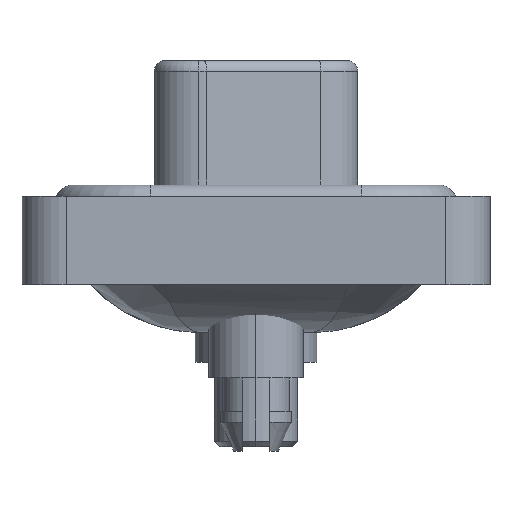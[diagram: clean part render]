
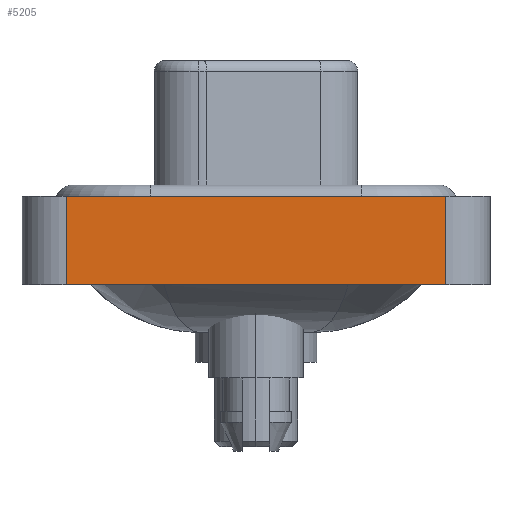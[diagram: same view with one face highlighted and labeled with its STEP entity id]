
A CAD part, left-side view. The second image highlights one B-rep face of the part: STEP entity #5205.
In plain terms, the highlighted planar face has unit normal (-1, 0, 0).
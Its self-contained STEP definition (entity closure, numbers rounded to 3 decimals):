
#461 = ORIENTED_EDGE ( 'NONE', *, *, #5446, .T. ) ;
#1047 = LINE ( 'NONE', #12623, #9949 ) ;
#2676 = LINE ( 'NONE', #12589, #4249 ) ;
#2811 = EDGE_CURVE ( 'NONE', #2993, #15523, #12068, .T. ) ;
#2993 = VERTEX_POINT ( 'NONE', #5460 ) ;
#4249 = VECTOR ( 'NONE', #14077, 1000. ) ;
#4266 = ORIENTED_EDGE ( 'NONE', *, *, #16483, .F. ) ;
#4294 = ORIENTED_EDGE ( 'NONE', *, *, #2811, .F. ) ;
#4490 = VERTEX_POINT ( 'NONE', #11666 ) ;
#4779 = ORIENTED_EDGE ( 'NONE', *, *, #6133, .T. ) ;
#5205 = ADVANCED_FACE ( 'NONE', ( #11688 ), #11243, .T. ) ;
#5334 = VERTEX_POINT ( 'NONE', #11087 ) ;
#5446 = EDGE_CURVE ( 'NONE', #4490, #15523, #2676, .T. ) ;
#5460 = CARTESIAN_POINT ( 'NONE',  ( -7.25, 8.55, 0.4 ) ) ;
#5566 = EDGE_LOOP ( 'NONE', ( #461, #4294, #4266, #4779 ) ) ;
#6133 = EDGE_CURVE ( 'NONE', #5334, #4490, #17828, .T. ) ;
#6440 = VECTOR ( 'NONE', #17737, 1000. ) ;
#7763 = CARTESIAN_POINT ( 'NONE',  ( -7.25, -8.55, -3.6 ) ) ;
#8317 = DIRECTION ( 'NONE',  ( 0., 0., 1. ) ) ;
#9949 = VECTOR ( 'NONE', #12258, 1000. ) ;
#10236 = CARTESIAN_POINT ( 'NONE',  ( -7.25, -8.55, 0.4 ) ) ;
#10419 = VECTOR ( 'NONE', #10669, 1000. ) ;
#10669 = DIRECTION ( 'NONE',  ( 0., -1., 0. ) ) ;
#11087 = CARTESIAN_POINT ( 'NONE',  ( -7.25, 8.55, -3.6 ) ) ;
#11243 = PLANE ( 'NONE',  #16892 ) ;
#11666 = CARTESIAN_POINT ( 'NONE',  ( -7.25, -8.55, -3.6 ) ) ;
#11688 = FACE_OUTER_BOUND ( 'NONE', #5566, .T. ) ;
#12068 = LINE ( 'NONE', #17817, #10419 ) ;
#12258 = DIRECTION ( 'NONE',  ( 0., 0., 1. ) ) ;
#12589 = CARTESIAN_POINT ( 'NONE',  ( -7.25, -8.55, -3.6 ) ) ;
#12623 = CARTESIAN_POINT ( 'NONE',  ( -7.25, 8.55, -3.6 ) ) ;
#14077 = DIRECTION ( 'NONE',  ( 0., 0., 1. ) ) ;
#15523 = VERTEX_POINT ( 'NONE', #10236 ) ;
#16483 = EDGE_CURVE ( 'NONE', #5334, #2993, #1047, .T. ) ;
#16878 = DIRECTION ( 'NONE',  ( -1., 0., 0. ) ) ;
#16892 = AXIS2_PLACEMENT_3D ( 'NONE', #16983, #16878, #8317 ) ;
#16983 = CARTESIAN_POINT ( 'NONE',  ( -7.25, -8.55, -3.6 ) ) ;
#17737 = DIRECTION ( 'NONE',  ( 0., -1., 0. ) ) ;
#17817 = CARTESIAN_POINT ( 'NONE',  ( -7.25, -8.55, 0.4 ) ) ;
#17828 = LINE ( 'NONE', #7763, #6440 ) ;
